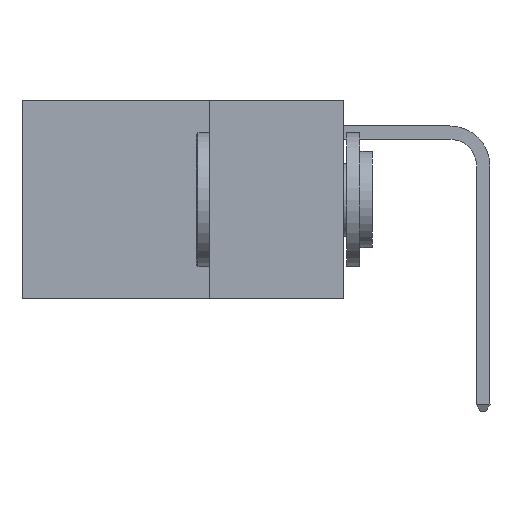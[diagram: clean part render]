
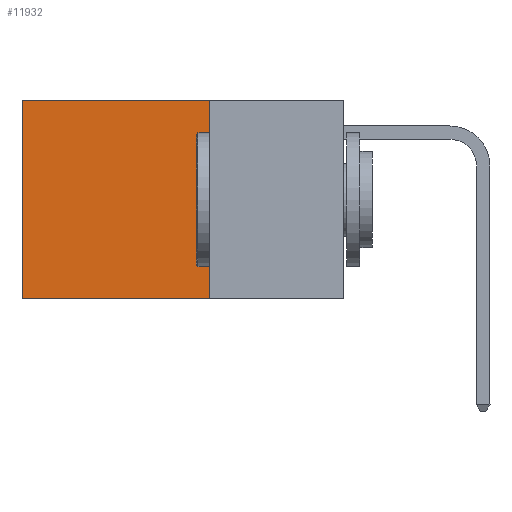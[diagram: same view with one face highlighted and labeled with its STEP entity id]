
A CAD part, left-side view. The second image highlights one B-rep face of the part: STEP entity #11932.
In plain terms, the highlighted planar face has unit normal (-1, 0, 0).
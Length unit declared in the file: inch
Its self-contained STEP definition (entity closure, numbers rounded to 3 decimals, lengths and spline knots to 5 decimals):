
#695 = FACE_OUTER_BOUND ( 'NONE', #11982, .T. ) ;
#2395 = CARTESIAN_POINT ( 'NONE',  ( 0.2625, 0.25, -0.37 ) ) ;
#2662 = EDGE_CURVE ( 'NONE', #10355, #5098, #8962, .T. ) ;
#3214 = PLANE ( 'NONE',  #13941 ) ;
#3271 = ORIENTED_EDGE ( 'NONE', *, *, #6902, .T. ) ;
#4951 = LINE ( 'NONE', #12506, #5468 ) ;
#5098 = VERTEX_POINT ( 'NONE', #6802 ) ;
#5397 = DIRECTION ( 'NONE',  ( 0., 0., -1. ) ) ;
#5468 = VECTOR ( 'NONE', #12677, 39.37008 ) ;
#5499 = VECTOR ( 'NONE', #13243, 39.37008 ) ;
#5545 = LINE ( 'NONE', #13192, #5499 ) ;
#5680 = CARTESIAN_POINT ( 'NONE',  ( 0.2625, 0.25, 0. ) ) ;
#5709 = CARTESIAN_POINT ( 'NONE',  ( 0.2625, 0.6, 0. ) ) ;
#5820 = CARTESIAN_POINT ( 'NONE',  ( 0.2625, 0.25, 0. ) ) ;
#6157 = LINE ( 'NONE', #13950, #6365 ) ;
#6365 = VECTOR ( 'NONE', #13918, 39.37008 ) ;
#6802 = CARTESIAN_POINT ( 'NONE',  ( 0.2625, 0.6, -0.37 ) ) ;
#6820 = EDGE_CURVE ( 'NONE', #15555, #5098, #6157, .T. ) ;
#6902 = EDGE_CURVE ( 'NONE', #13625, #10355, #5545, .T. ) ;
#6957 = EDGE_CURVE ( 'NONE', #13625, #15555, #4951, .T. ) ;
#7021 = DIRECTION ( 'NONE',  ( 1., 0., 0. ) ) ;
#8377 = VECTOR ( 'NONE', #5397, 39.37008 ) ;
#8962 = LINE ( 'NONE', #5709, #8377 ) ;
#10355 = VERTEX_POINT ( 'NONE', #11315 ) ;
#11315 = CARTESIAN_POINT ( 'NONE',  ( 0.2625, 0.6, 0. ) ) ;
#11932 = ADVANCED_FACE ( 'NONE', ( #695 ), #3214, .F. ) ;
#11982 = EDGE_LOOP ( 'NONE', ( #15202, #14274, #14149, #3271 ) ) ;
#12506 = CARTESIAN_POINT ( 'NONE',  ( 0.2625, 0.25, 0. ) ) ;
#12677 = DIRECTION ( 'NONE',  ( 0., 0., -1. ) ) ;
#13192 = CARTESIAN_POINT ( 'NONE',  ( 0.2625, 0.25, 0. ) ) ;
#13243 = DIRECTION ( 'NONE',  ( 0., 1., 0. ) ) ;
#13625 = VERTEX_POINT ( 'NONE', #5820 ) ;
#13918 = DIRECTION ( 'NONE',  ( 0., 1., 0. ) ) ;
#13941 = AXIS2_PLACEMENT_3D ( 'NONE', #5680, #7021, #15235 ) ;
#13950 = CARTESIAN_POINT ( 'NONE',  ( 0.2625, 0.25, -0.37 ) ) ;
#14149 = ORIENTED_EDGE ( 'NONE', *, *, #6957, .F. ) ;
#14274 = ORIENTED_EDGE ( 'NONE', *, *, #6820, .F. ) ;
#15202 = ORIENTED_EDGE ( 'NONE', *, *, #2662, .T. ) ;
#15235 = DIRECTION ( 'NONE',  ( 0., 0., -1. ) ) ;
#15555 = VERTEX_POINT ( 'NONE', #2395 ) ;
